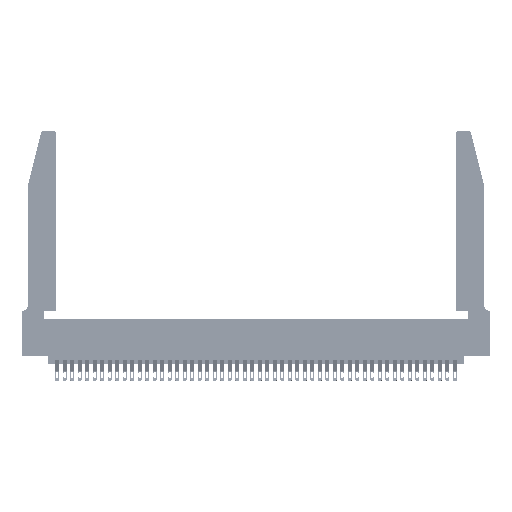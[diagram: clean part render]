
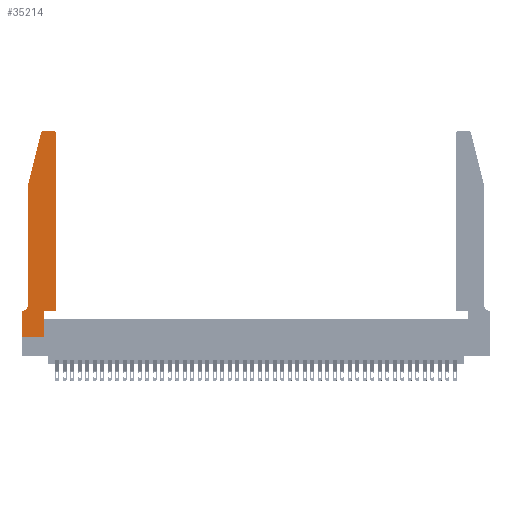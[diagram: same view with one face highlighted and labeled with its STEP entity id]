
A CAD part, top view. The second image highlights one B-rep face of the part: STEP entity #35214.
In plain terms, the highlighted planar face has unit normal (0, 0, 1).
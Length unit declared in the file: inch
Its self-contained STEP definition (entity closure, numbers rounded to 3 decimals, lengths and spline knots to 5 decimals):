
#452 = CIRCLE ( 'NONE', #4406, 0.03 ) ;
#572 = DIRECTION ( 'NONE',  ( 0., -1., 0. ) ) ;
#1071 = DIRECTION ( 'NONE',  ( -0.239, -0.971, 0. ) ) ;
#2169 = CARTESIAN_POINT ( 'NONE',  ( 0.4505, 2.72, 0.37 ) ) ;
#3402 = CARTESIAN_POINT ( 'NONE',  ( 0.4505, 0.35, 0.37 ) ) ;
#3790 = CARTESIAN_POINT ( 'NONE',  ( 0.284, 2.75, 0.37 ) ) ;
#4141 = VERTEX_POINT ( 'NONE', #42455 ) ;
#4380 = VECTOR ( 'NONE', #19286, 39.37008 ) ;
#4396 = LINE ( 'NONE', #22525, #42695 ) ;
#4406 = AXIS2_PLACEMENT_3D ( 'NONE', #41289, #16565, #27441 ) ;
#4551 = VERTEX_POINT ( 'NONE', #24992 ) ;
#6084 = AXIS2_PLACEMENT_3D ( 'NONE', #30501, #30349, #20051 ) ;
#6380 = ORIENTED_EDGE ( 'NONE', *, *, #31760, .T. ) ;
#7156 = VECTOR ( 'NONE', #37933, 39.37008 ) ;
#7434 = ORIENTED_EDGE ( 'NONE', *, *, #40315, .T. ) ;
#7513 = CARTESIAN_POINT ( 'NONE',  ( 0.0055, 0.35, 0.37 ) ) ;
#7933 = ORIENTED_EDGE ( 'NONE', *, *, #32181, .T. ) ;
#8446 = ORIENTED_EDGE ( 'NONE', *, *, #20721, .T. ) ;
#9037 = DIRECTION ( 'NONE',  ( 0., 0., 1. ) ) ;
#9081 = CARTESIAN_POINT ( 'NONE',  ( 0., 0., 0.37 ) ) ;
#10038 = DIRECTION ( 'NONE',  ( -1., 0., 0. ) ) ;
#11117 = LINE ( 'NONE', #11454, #23873 ) ;
#11454 = CARTESIAN_POINT ( 'NONE',  ( 0.0755, 2., 0.37 ) ) ;
#12446 = EDGE_LOOP ( 'NONE', ( #20308, #43089, #7933, #18594, #25014, #37409, #33767, #7434, #6380, #26302, #17561, #8446 ) ) ;
#12898 = PLANE ( 'NONE',  #6084 ) ;
#12917 = CARTESIAN_POINT ( 'NONE',  ( 0.0055, 0.42, 0.37 ) ) ;
#13798 = LINE ( 'NONE', #19121, #4380 ) ;
#15188 = EDGE_CURVE ( 'NONE', #15822, #19731, #23533, .T. ) ;
#15211 = FACE_OUTER_BOUND ( 'NONE', #12446, .T. ) ;
#15822 = VERTEX_POINT ( 'NONE', #24949 ) ;
#15867 = EDGE_CURVE ( 'NONE', #33163, #4551, #34052, .T. ) ;
#15868 = CIRCLE ( 'NONE', #28868, 0.03 ) ;
#16031 = EDGE_CURVE ( 'NONE', #39528, #44437, #37725, .T. ) ;
#16565 = DIRECTION ( 'NONE',  ( 0., 0., 1. ) ) ;
#16570 = VERTEX_POINT ( 'NONE', #7513 ) ;
#16744 = VECTOR ( 'NONE', #25269, 39.37008 ) ;
#17560 = DIRECTION ( 'NONE',  ( -1., 0., 0. ) ) ;
#17561 = ORIENTED_EDGE ( 'NONE', *, *, #23222, .T. ) ;
#18594 = ORIENTED_EDGE ( 'NONE', *, *, #30893, .T. ) ;
#18779 = DIRECTION ( 'NONE',  ( 0., 1., 0. ) ) ;
#19121 = CARTESIAN_POINT ( 'NONE',  ( 0., 0., 0.37 ) ) ;
#19286 = DIRECTION ( 'NONE',  ( 1., 0., 0. ) ) ;
#19731 = VERTEX_POINT ( 'NONE', #3790 ) ;
#20051 = DIRECTION ( 'NONE',  ( 1., 0., 0. ) ) ;
#20308 = ORIENTED_EDGE ( 'NONE', *, *, #15188, .T. ) ;
#20721 = EDGE_CURVE ( 'NONE', #23983, #15822, #452, .T. ) ;
#22088 = CARTESIAN_POINT ( 'NONE',  ( 0.2865, 0., 0.37 ) ) ;
#22435 = VECTOR ( 'NONE', #17560, 39.37008 ) ;
#22525 = CARTESIAN_POINT ( 'NONE',  ( 0.2865, 0.35, 0.37 ) ) ;
#23222 = EDGE_CURVE ( 'NONE', #4551, #23983, #45985, .T. ) ;
#23533 = LINE ( 'NONE', #35445, #22435 ) ;
#23873 = VECTOR ( 'NONE', #572, 39.37008 ) ;
#23983 = VERTEX_POINT ( 'NONE', #2169 ) ;
#24949 = CARTESIAN_POINT ( 'NONE',  ( 0.4205, 2.75, 0.37 ) ) ;
#24992 = CARTESIAN_POINT ( 'NONE',  ( 0.4505, 0.35, 0.37 ) ) ;
#25014 = ORIENTED_EDGE ( 'NONE', *, *, #25462, .T. ) ;
#25269 = DIRECTION ( 'NONE',  ( 1., 0., 0. ) ) ;
#25462 = EDGE_CURVE ( 'NONE', #4141, #16570, #45870, .T. ) ;
#26120 = VERTEX_POINT ( 'NONE', #40836 ) ;
#26302 = ORIENTED_EDGE ( 'NONE', *, *, #15867, .T. ) ;
#26462 = DIRECTION ( 'NONE',  ( 0., 0., -1. ) ) ;
#26765 = DIRECTION ( 'NONE',  ( -1., 0., 0. ) ) ;
#27078 = CARTESIAN_POINT ( 'NONE',  ( 0.2865, 0.35, 0.37 ) ) ;
#27311 = VERTEX_POINT ( 'NONE', #22088 ) ;
#27441 = DIRECTION ( 'NONE',  ( 1., 0., 0. ) ) ;
#27634 = VECTOR ( 'NONE', #33169, 39.37008 ) ;
#27676 = VECTOR ( 'NONE', #1071, 39.37008 ) ;
#28817 = LINE ( 'NONE', #36028, #27676 ) ;
#28868 = AXIS2_PLACEMENT_3D ( 'NONE', #33292, #9037, #40398 ) ;
#30349 = DIRECTION ( 'NONE',  ( 0., 0., 1. ) ) ;
#30501 = CARTESIAN_POINT ( 'NONE',  ( 0., 0.35, 0.37 ) ) ;
#30893 = EDGE_CURVE ( 'NONE', #39574, #4141, #11117, .T. ) ;
#31760 = EDGE_CURVE ( 'NONE', #27311, #33163, #4396, .T. ) ;
#32181 = EDGE_CURVE ( 'NONE', #26120, #39574, #28817, .T. ) ;
#33163 = VERTEX_POINT ( 'NONE', #27078 ) ;
#33169 = DIRECTION ( 'NONE',  ( 0., 1., 0. ) ) ;
#33292 = CARTESIAN_POINT ( 'NONE',  ( 0.284, 2.72, 0.37 ) ) ;
#33767 = ORIENTED_EDGE ( 'NONE', *, *, #16031, .T. ) ;
#34052 = LINE ( 'NONE', #3402, #16744 ) ;
#34895 = CARTESIAN_POINT ( 'NONE',  ( 0.0755, 0.35, 0.37 ) ) ;
#35214 = ADVANCED_FACE ( 'NONE', ( #15211 ), #12898, .T. ) ;
#35445 = CARTESIAN_POINT ( 'NONE',  ( 0.2605, 2.75, 0.37 ) ) ;
#36028 = CARTESIAN_POINT ( 'NONE',  ( 0.0755, 2., 0.37 ) ) ;
#36277 = CARTESIAN_POINT ( 'NONE',  ( 0., 0.35, 0.37 ) ) ;
#36596 = EDGE_CURVE ( 'NONE', #16570, #39528, #38102, .T. ) ;
#37409 = ORIENTED_EDGE ( 'NONE', *, *, #36596, .T. ) ;
#37725 = LINE ( 'NONE', #9081, #7156 ) ;
#37933 = DIRECTION ( 'NONE',  ( 0., -1., 0. ) ) ;
#38102 = LINE ( 'NONE', #34895, #43075 ) ;
#39528 = VERTEX_POINT ( 'NONE', #36277 ) ;
#39574 = VERTEX_POINT ( 'NONE', #40149 ) ;
#40149 = CARTESIAN_POINT ( 'NONE',  ( 0.0755, 2., 0.37 ) ) ;
#40283 = CARTESIAN_POINT ( 'NONE',  ( 0.4505, 0.35, 0.37 ) ) ;
#40315 = EDGE_CURVE ( 'NONE', #44437, #27311, #13798, .T. ) ;
#40398 = DIRECTION ( 'NONE',  ( 1., 0., 0. ) ) ;
#40836 = CARTESIAN_POINT ( 'NONE',  ( 0.25487, 2.72718, 0.37 ) ) ;
#41151 = AXIS2_PLACEMENT_3D ( 'NONE', #12917, #26462, #26765 ) ;
#41289 = CARTESIAN_POINT ( 'NONE',  ( 0.4205, 2.72, 0.37 ) ) ;
#41810 = EDGE_CURVE ( 'NONE', #19731, #26120, #15868, .T. ) ;
#42455 = CARTESIAN_POINT ( 'NONE',  ( 0.0755, 0.42, 0.37 ) ) ;
#42695 = VECTOR ( 'NONE', #18779, 39.37008 ) ;
#43075 = VECTOR ( 'NONE', #10038, 39.37008 ) ;
#43089 = ORIENTED_EDGE ( 'NONE', *, *, #41810, .T. ) ;
#43995 = CARTESIAN_POINT ( 'NONE',  ( 0., 0., 0.37 ) ) ;
#44437 = VERTEX_POINT ( 'NONE', #43995 ) ;
#45870 = CIRCLE ( 'NONE', #41151, 0.07 ) ;
#45985 = LINE ( 'NONE', #40283, #27634 ) ;
